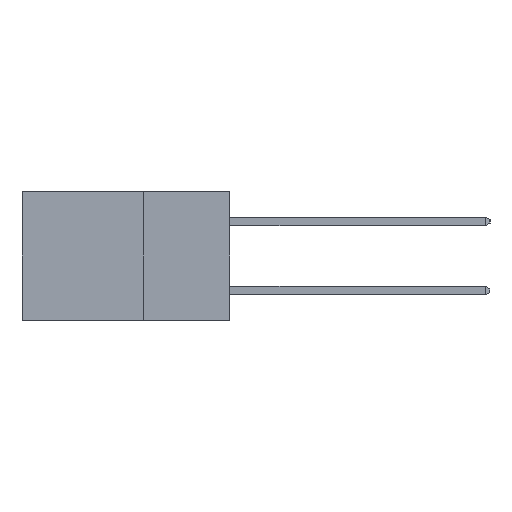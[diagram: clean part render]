
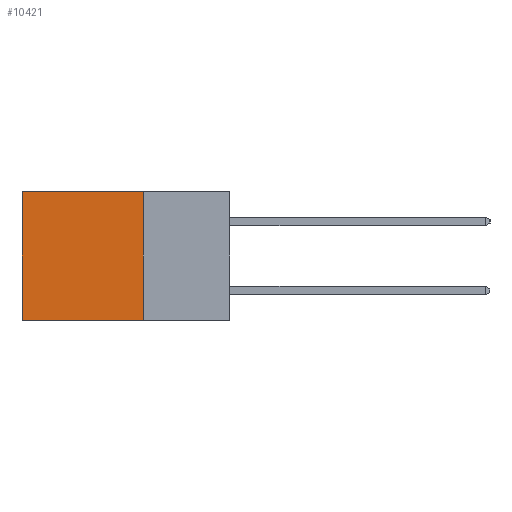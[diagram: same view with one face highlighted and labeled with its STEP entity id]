
A CAD part, left-side view. The second image highlights one B-rep face of the part: STEP entity #10421.
In plain terms, the highlighted planar face has unit normal (-1, 0, 0).
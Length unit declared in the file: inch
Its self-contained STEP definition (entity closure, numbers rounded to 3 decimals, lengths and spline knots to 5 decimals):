
#638 = DIRECTION ( 'NONE',  ( 0., 1., 0. ) ) ;
#1739 = CARTESIAN_POINT ( 'NONE',  ( 0.298, 0.6, 0. ) ) ;
#2078 = EDGE_CURVE ( 'NONE', #4474, #21247, #11446, .T. ) ;
#3822 = AXIS2_PLACEMENT_3D ( 'NONE', #10317, #22036, #12006 ) ;
#4456 = LINE ( 'NONE', #5310, #9085 ) ;
#4474 = VERTEX_POINT ( 'NONE', #1739 ) ;
#5310 = CARTESIAN_POINT ( 'NONE',  ( 0.298, 0.25, -0.37 ) ) ;
#5754 = DIRECTION ( 'NONE',  ( 0., 0., -1. ) ) ;
#5755 = EDGE_CURVE ( 'NONE', #20313, #21247, #4456, .T. ) ;
#6822 = VECTOR ( 'NONE', #9577, 39.37008 ) ;
#8556 = ORIENTED_EDGE ( 'NONE', *, *, #2078, .T. ) ;
#9085 = VECTOR ( 'NONE', #15573, 39.37008 ) ;
#9493 = ORIENTED_EDGE ( 'NONE', *, *, #18288, .F. ) ;
#9527 = VECTOR ( 'NONE', #638, 39.37008 ) ;
#9577 = DIRECTION ( 'NONE',  ( 0., 0., -1. ) ) ;
#10317 = CARTESIAN_POINT ( 'NONE',  ( 0.298, 0.25, 0. ) ) ;
#10421 = ADVANCED_FACE ( 'NONE', ( #14077 ), #18726, .F. ) ;
#11122 = VERTEX_POINT ( 'NONE', #14926 ) ;
#11446 = LINE ( 'NONE', #12111, #6822 ) ;
#12006 = DIRECTION ( 'NONE',  ( 0., 0., -1. ) ) ;
#12111 = CARTESIAN_POINT ( 'NONE',  ( 0.298, 0.6, 0. ) ) ;
#12143 = VECTOR ( 'NONE', #5754, 39.37008 ) ;
#12676 = LINE ( 'NONE', #14315, #12143 ) ;
#12716 = CARTESIAN_POINT ( 'NONE',  ( 0.298, 0.25, 0. ) ) ;
#14077 = FACE_OUTER_BOUND ( 'NONE', #18896, .T. ) ;
#14315 = CARTESIAN_POINT ( 'NONE',  ( 0.298, 0.25, 0. ) ) ;
#14926 = CARTESIAN_POINT ( 'NONE',  ( 0.298, 0.25, 0. ) ) ;
#15573 = DIRECTION ( 'NONE',  ( 0., 1., 0. ) ) ;
#17112 = ORIENTED_EDGE ( 'NONE', *, *, #5755, .F. ) ;
#17383 = CARTESIAN_POINT ( 'NONE',  ( 0.298, 0.6, -0.37 ) ) ;
#17610 = EDGE_CURVE ( 'NONE', #11122, #4474, #21867, .T. ) ;
#17685 = ORIENTED_EDGE ( 'NONE', *, *, #17610, .T. ) ;
#18288 = EDGE_CURVE ( 'NONE', #11122, #20313, #12676, .T. ) ;
#18726 = PLANE ( 'NONE',  #3822 ) ;
#18896 = EDGE_LOOP ( 'NONE', ( #8556, #17112, #9493, #17685 ) ) ;
#20313 = VERTEX_POINT ( 'NONE', #21769 ) ;
#21247 = VERTEX_POINT ( 'NONE', #17383 ) ;
#21769 = CARTESIAN_POINT ( 'NONE',  ( 0.298, 0.25, -0.37 ) ) ;
#21867 = LINE ( 'NONE', #12716, #9527 ) ;
#22036 = DIRECTION ( 'NONE',  ( 1., 0., 0. ) ) ;
